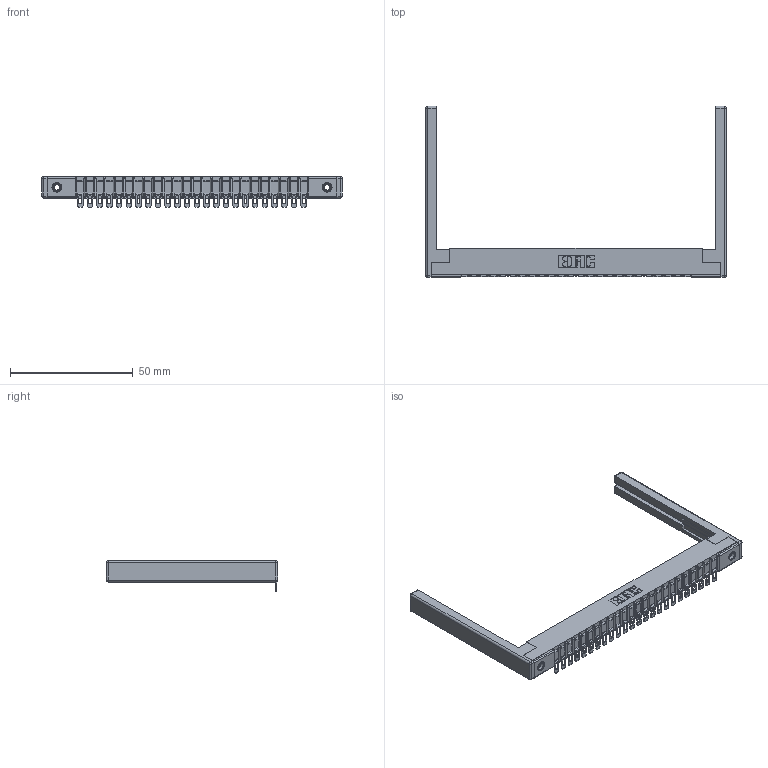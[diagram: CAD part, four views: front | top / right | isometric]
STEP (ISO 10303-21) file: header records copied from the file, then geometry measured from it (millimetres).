
FILE_DESCRIPTION (( 'STEP AP203' ), '1' );
FILE_NAME ('307-024-554-168.STEP', '2019-09-05T01:13:08', ( '' ), ( '' ), 'SwSTEP 2.0', 'SolidWorks 2016', '' );
FILE_SCHEMA (( 'CONFIG_CONTROL_DESIGN' ));
Length unit declared in the file: inch
Products named in the file (5): 307-290-002_554; 307 Part_.156 Dia Mounting Holes; 307-024-554-168; 345-250-001_345-250-001-102; 307-220-068
Assembly tree (29 placements, depth 2):
  307-024-554-168
    307 Part_.156 Dia Mounting Holes
    307-290-002_554  x24
    307-220-068  x2
    345-250-001_345-250-001-102  x2
Bounding box: 122.53 x 69.98 x 12.52 mm (x, y, z)
Volume: 12657.6 mm3; surface area: 18961 mm2
Topology: 29 solids, 29 shells, 2241 faces, 6785 edges, 4434 vertices
Faces by surface type: plane 1262, cylinder 905, sphere 58, cone 12, torus 4
Entity records: 26518 total; most frequent: CARTESIAN_POINT 4435, ORIENTED_EDGE 4414, DIRECTION 4341, EDGE_CURVE 2207, VECTOR 1673, LINE 1673, VERTEX_POINT 1428, AXIS2_PLACEMENT_3D 1334
